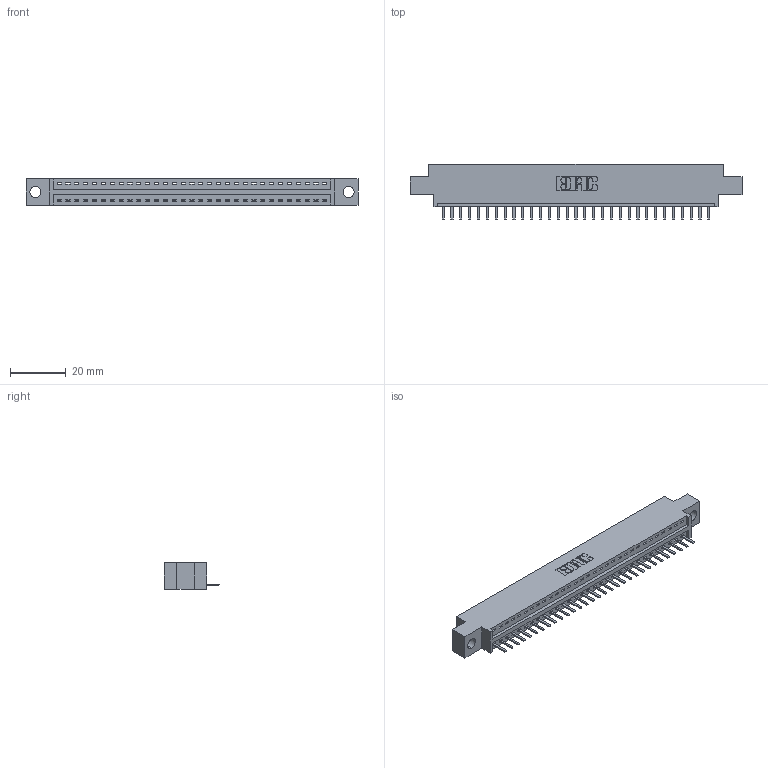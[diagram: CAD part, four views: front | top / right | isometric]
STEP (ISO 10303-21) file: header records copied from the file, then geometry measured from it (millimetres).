
FILE_DESCRIPTION (( 'STEP AP203' ), '1' );
FILE_NAME ('346-031-520-604.STEP', '2022-05-06T16:33:56', ( '' ), ( '' ), 'SwSTEP 2.0', 'SolidWorks 2020', '' );
FILE_SCHEMA (( 'CONFIG_CONTROL_DESIGN' ));
Length unit declared in the file: inch
Products named in the file (3): 346 Part_0.170 Offset - 0.156 Dia-TH; 346-031-520-604; 345-292-001_345-293-120
Assembly tree (32 placements, depth 2):
  346-031-520-604
    346 Part_0.170 Offset - 0.156 Dia-TH
    345-292-001_345-293-120  x31
Bounding box: 119 x 20.02 x 9.4 mm (x, y, z)
Volume: 10965.3 mm3; surface area: 13286.5 mm2
Topology: 32 solids, 32 shells, 2062 faces, 6081 edges, 3970 vertices
Faces by surface type: plane 1396, cylinder 666
Entity records: 21385 total; most frequent: CARTESIAN_POINT 3691, ORIENTED_EDGE 3642, DIRECTION 3255, EDGE_CURVE 1821, LINE 1561, VECTOR 1561, VERTEX_POINT 1210, AXIS2_PLACEMENT_3D 847
